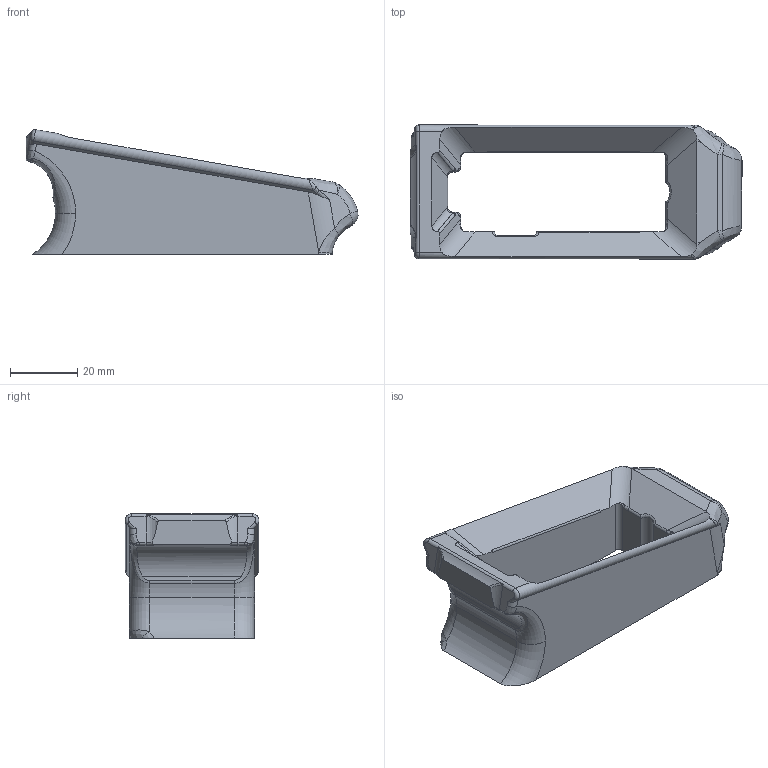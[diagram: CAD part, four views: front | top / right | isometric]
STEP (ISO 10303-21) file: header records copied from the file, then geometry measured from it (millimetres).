
FILE_DESCRIPTION (( 'STEP AP214' ), '1' );
FILE_NAME ('Magwell_3a.STEP', '2015-10-23T19:40:46', ( 'WarFairy' ), ( '' ), 'SwSTEP 2.0', 'SolidWorks 2015', '' );
FILE_SCHEMA (( 'AUTOMOTIVE_DESIGN' ));
Length unit declared in the file: millimetre
Products named in the file (1): Magwell_3a
Bounding box: 98.58 x 39.78 x 37.04 mm (x, y, z)
Volume: 44003.1 mm3; surface area: 15514.8 mm2
Topology: 1 solids, 1 shells, 181 faces, 472 edges, 287 vertices
Faces by surface type: bspline 64, cylinder 53, plane 46, torus 11, sphere 7
Entity records: 8236 total; most frequent: CARTESIAN_POINT 4419, ORIENTED_EDGE 934, DIRECTION 615, EDGE_CURVE 467, VERTEX_POINT 287, AXIS2_PLACEMENT_3D 227, EDGE_LOOP 182, FACE_OUTER_BOUND 181
